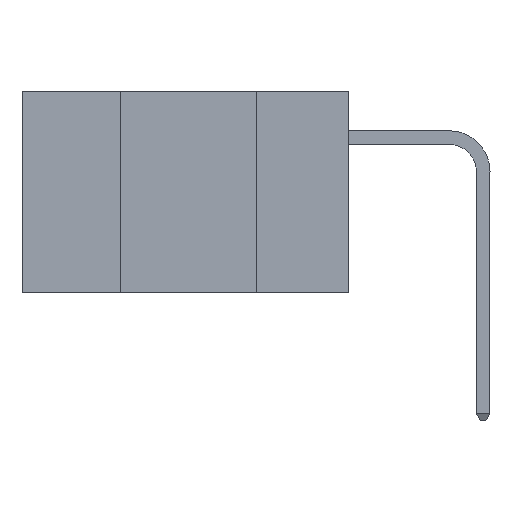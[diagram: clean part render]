
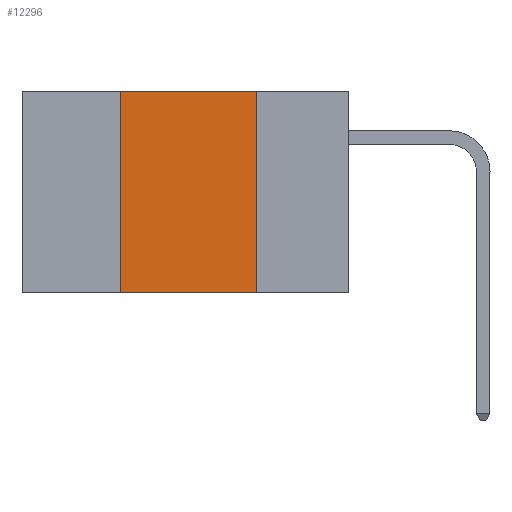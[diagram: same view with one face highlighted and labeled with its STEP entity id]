
A CAD part, left-side view. The second image highlights one B-rep face of the part: STEP entity #12296.
In plain terms, the highlighted planar face has unit normal (-1, 0, 0).
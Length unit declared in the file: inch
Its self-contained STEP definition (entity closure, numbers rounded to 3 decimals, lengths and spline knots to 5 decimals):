
#370 = CARTESIAN_POINT ( 'NONE',  ( 0., 0.17, 0. ) ) ;
#958 = EDGE_CURVE ( 'NONE', #8513, #13919, #23775, .T. ) ;
#1428 = VECTOR ( 'NONE', #5978, 39.37008 ) ;
#2009 = CARTESIAN_POINT ( 'NONE',  ( 0., 0.6, 0. ) ) ;
#2404 = CARTESIAN_POINT ( 'NONE',  ( 0., 0.17, 0. ) ) ;
#3320 = VERTEX_POINT ( 'NONE', #6053 ) ;
#5978 = DIRECTION ( 'NONE',  ( 0., -1., 0. ) ) ;
#6053 = CARTESIAN_POINT ( 'NONE',  ( 0., 0.17, -0.37 ) ) ;
#6151 = PLANE ( 'NONE',  #7773 ) ;
#7773 = AXIS2_PLACEMENT_3D ( 'NONE', #2009, #20226, #8170 ) ;
#8170 = DIRECTION ( 'NONE',  ( 0., 0., -1. ) ) ;
#8178 = VECTOR ( 'NONE', #18609, 39.37008 ) ;
#8513 = VERTEX_POINT ( 'NONE', #20228 ) ;
#9505 = CARTESIAN_POINT ( 'NONE',  ( 0., 0.42, 0. ) ) ;
#10162 = DIRECTION ( 'NONE',  ( 0., 0., 1. ) ) ;
#11745 = VERTEX_POINT ( 'NONE', #2404 ) ;
#12146 = DIRECTION ( 'NONE',  ( 0., -1., 0. ) ) ;
#12256 = LINE ( 'NONE', #26047, #1428 ) ;
#12275 = EDGE_CURVE ( 'NONE', #8513, #3320, #12722, .T. ) ;
#12296 = ADVANCED_FACE ( 'NONE', ( #17505 ), #6151, .F. ) ;
#12722 = LINE ( 'NONE', #22167, #18111 ) ;
#12908 = LINE ( 'NONE', #370, #8178 ) ;
#13133 = ORIENTED_EDGE ( 'NONE', *, *, #12275, .T. ) ;
#13919 = VERTEX_POINT ( 'NONE', #9505 ) ;
#17505 = FACE_OUTER_BOUND ( 'NONE', #18690, .T. ) ;
#18111 = VECTOR ( 'NONE', #12146, 39.37008 ) ;
#18415 = VECTOR ( 'NONE', #10162, 39.37008 ) ;
#18609 = DIRECTION ( 'NONE',  ( 0., 0., -1. ) ) ;
#18690 = EDGE_LOOP ( 'NONE', ( #21932, #24504, #21987, #13133 ) ) ;
#20226 = DIRECTION ( 'NONE',  ( 1., 0., 0. ) ) ;
#20228 = CARTESIAN_POINT ( 'NONE',  ( 0., 0.42, -0.37 ) ) ;
#21932 = ORIENTED_EDGE ( 'NONE', *, *, #24072, .F. ) ;
#21933 = CARTESIAN_POINT ( 'NONE',  ( 0., 0.42, 0. ) ) ;
#21987 = ORIENTED_EDGE ( 'NONE', *, *, #958, .F. ) ;
#22167 = CARTESIAN_POINT ( 'NONE',  ( 0., 0.6, -0.37 ) ) ;
#23775 = LINE ( 'NONE', #21933, #18415 ) ;
#24072 = EDGE_CURVE ( 'NONE', #11745, #3320, #12908, .T. ) ;
#24504 = ORIENTED_EDGE ( 'NONE', *, *, #24523, .F. ) ;
#24523 = EDGE_CURVE ( 'NONE', #13919, #11745, #12256, .T. ) ;
#26047 = CARTESIAN_POINT ( 'NONE',  ( 0., 0.6, 0. ) ) ;
